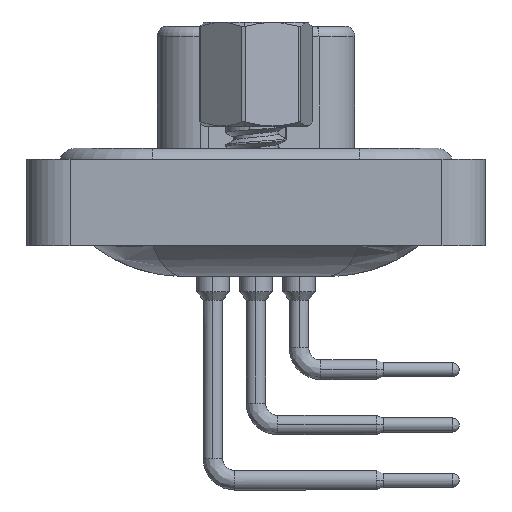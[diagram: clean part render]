
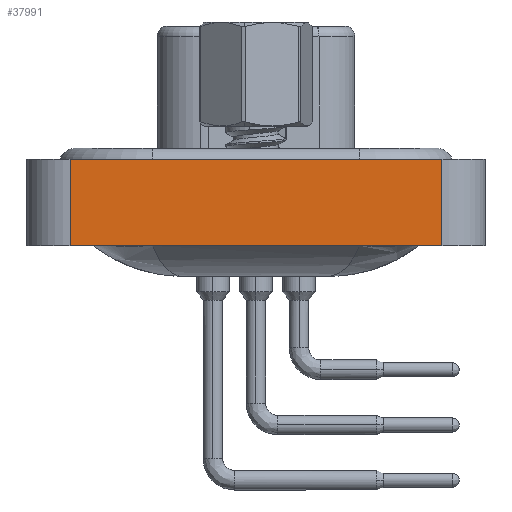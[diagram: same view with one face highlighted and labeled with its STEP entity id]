
A CAD part, left-side view. The second image highlights one B-rep face of the part: STEP entity #37991.
In plain terms, the highlighted planar face has unit normal (-1, 0, 0).
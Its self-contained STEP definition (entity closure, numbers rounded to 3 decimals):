
#665 = DIRECTION ( 'NONE',  ( 0., -1., 0. ) ) ;
#890 = CARTESIAN_POINT ( 'NONE',  ( -7.35, -8.55, -3.6 ) ) ;
#909 = LINE ( 'NONE', #40229, #4888 ) ;
#1034 = CARTESIAN_POINT ( 'NONE',  ( -7.35, -8.55, -3.6 ) ) ;
#1100 = LINE ( 'NONE', #890, #20981 ) ;
#1945 = CARTESIAN_POINT ( 'NONE',  ( -7.35, -8.55, -3.6 ) ) ;
#3322 = VECTOR ( 'NONE', #7694, 1000. ) ;
#3640 = EDGE_LOOP ( 'NONE', ( #30170, #14781, #9683, #31021 ) ) ;
#4389 = VERTEX_POINT ( 'NONE', #35679 ) ;
#4888 = VECTOR ( 'NONE', #40887, 1000. ) ;
#5766 = EDGE_CURVE ( 'NONE', #4389, #16921, #909, .T. ) ;
#7694 = DIRECTION ( 'NONE',  ( 0., 0., 1. ) ) ;
#7750 = DIRECTION ( 'NONE',  ( -1., 0., 0. ) ) ;
#8238 = LINE ( 'NONE', #1945, #26086 ) ;
#9683 = ORIENTED_EDGE ( 'NONE', *, *, #16946, .F. ) ;
#9954 = VERTEX_POINT ( 'NONE', #21247 ) ;
#14667 = DIRECTION ( 'NONE',  ( 0., 0., 1. ) ) ;
#14781 = ORIENTED_EDGE ( 'NONE', *, *, #5766, .F. ) ;
#14875 = PLANE ( 'NONE',  #37125 ) ;
#16921 = VERTEX_POINT ( 'NONE', #36839 ) ;
#16946 = EDGE_CURVE ( 'NONE', #20282, #4389, #40525, .T. ) ;
#20282 = VERTEX_POINT ( 'NONE', #41186 ) ;
#20981 = VECTOR ( 'NONE', #665, 1000. ) ;
#21247 = CARTESIAN_POINT ( 'NONE',  ( -7.35, -8.55, -3.6 ) ) ;
#23690 = EDGE_CURVE ( 'NONE', #20282, #9954, #1100, .T. ) ;
#23899 = CARTESIAN_POINT ( 'NONE',  ( -7.35, 8.55, -3.6 ) ) ;
#26086 = VECTOR ( 'NONE', #34585, 1000. ) ;
#30170 = ORIENTED_EDGE ( 'NONE', *, *, #37458, .T. ) ;
#31021 = ORIENTED_EDGE ( 'NONE', *, *, #23690, .T. ) ;
#34321 = FACE_OUTER_BOUND ( 'NONE', #3640, .T. ) ;
#34585 = DIRECTION ( 'NONE',  ( 0., 0., 1. ) ) ;
#35679 = CARTESIAN_POINT ( 'NONE',  ( -7.35, 8.55, 0.4 ) ) ;
#36839 = CARTESIAN_POINT ( 'NONE',  ( -7.35, -8.55, 0.4 ) ) ;
#37125 = AXIS2_PLACEMENT_3D ( 'NONE', #1034, #7750, #14667 ) ;
#37458 = EDGE_CURVE ( 'NONE', #9954, #16921, #8238, .T. ) ;
#37991 = ADVANCED_FACE ( 'NONE', ( #34321 ), #14875, .T. ) ;
#40229 = CARTESIAN_POINT ( 'NONE',  ( -7.35, -8.55, 0.4 ) ) ;
#40525 = LINE ( 'NONE', #23899, #3322 ) ;
#40887 = DIRECTION ( 'NONE',  ( 0., -1., 0. ) ) ;
#41186 = CARTESIAN_POINT ( 'NONE',  ( -7.35, 8.55, -3.6 ) ) ;
